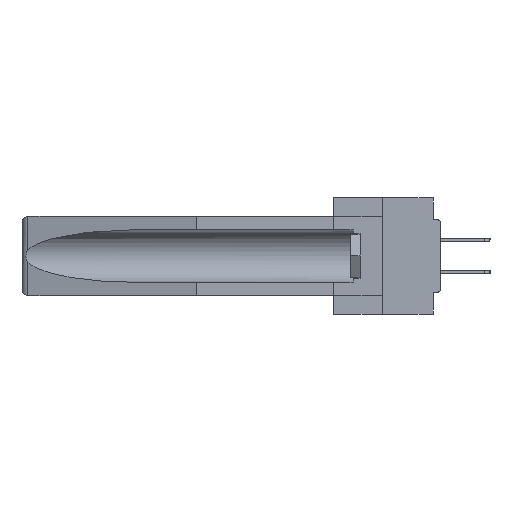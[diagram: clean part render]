
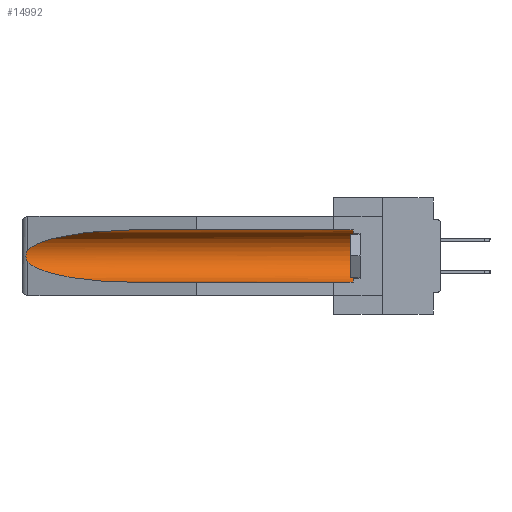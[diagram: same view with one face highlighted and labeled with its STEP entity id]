
A CAD part, left-side view. The second image highlights one B-rep face of the part: STEP entity #14992.
In plain terms, the highlighted cylindrical face has radius 2.857 mm (diameter 5.715 mm), a partial arc.
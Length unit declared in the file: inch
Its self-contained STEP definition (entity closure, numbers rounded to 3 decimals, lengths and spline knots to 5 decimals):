
#111 = VERTEX_POINT ( 'NONE', #24628 ) ;
#207 = VECTOR ( 'NONE', #23239, 39.37008 ) ;
#269 = CARTESIAN_POINT ( 'NONE',  ( 0.155, 1.07973, -0.284 ) ) ;
#1505 = LINE ( 'NONE', #4396, #2415 ) ;
#2100 = ORIENTED_EDGE ( 'NONE', *, *, #27193, .F. ) ;
#2415 = VECTOR ( 'NONE', #7474, 39.37008 ) ;
#3711 = CARTESIAN_POINT ( 'NONE',  ( 0.25451, 1.48313, -0.24835 ) ) ;
#3872 = ORIENTED_EDGE ( 'NONE', *, *, #9727, .T. ) ;
#4396 = CARTESIAN_POINT ( 'NONE',  ( 0.155, -0.30754, -0.059 ) ) ;
#4948 = CARTESIAN_POINT ( 'NONE',  ( 0.2675, 1.53308, -0.16763 ) ) ;
#5021 = VERTEX_POINT ( 'NONE', #32688 ) ;
#6171 = CYLINDRICAL_SURFACE ( 'NONE', #29870, 0.1125 ) ;
#6423 = CARTESIAN_POINT ( 'NONE',  ( 0.21114, 1.30732, -0.284 ) ) ;
#6682 = LINE ( 'NONE', #29462, #207 ) ;
#6717 = DIRECTION ( 'NONE',  ( 0., -1., 0. ) ) ;
#7474 = DIRECTION ( 'NONE',  ( 0., 1., 0. ) ) ;
#8298 = VERTEX_POINT ( 'NONE', #269 ) ;
#9727 = EDGE_CURVE ( 'NONE', #20303, #17446, #24305, .T. ) ;
#10373 = CARTESIAN_POINT ( 'NONE',  ( 0.26537, 1.52718, -0.19328 ) ) ;
#11486 = DIRECTION ( 'NONE',  ( 0., 0., 1. ) ) ;
#11732 = AXIS2_PLACEMENT_3D ( 'NONE', #24704, #6717, #22500 ) ;
#12064 = CARTESIAN_POINT ( 'NONE',  ( 0.155, 1.07973, -0.284 ) ) ;
#13337 = CARTESIAN_POINT ( 'NONE',  ( 0.26597, 1.52961, -0.15275 ) ) ;
#13363 = CARTESIAN_POINT ( 'NONE',  ( 0.21114, 1.30732, -0.059 ) ) ;
#13642 = CARTESIAN_POINT ( 'NONE',  ( 0.155, 0.126, -0.059 ) ) ;
#13966 = CARTESIAN_POINT ( 'NONE',  ( 0.26537, 1.52718, -0.19328 ) ) ;
#14992 = ADVANCED_FACE ( 'NONE', ( #31462 ), #6171, .F. ) ;
#15349 =( BOUNDED_CURVE ( )  B_SPLINE_CURVE ( 3, ( #18247, #13363, #36977, #19280 ),
 .UNSPECIFIED., .F., .F. ) 
 B_SPLINE_CURVE_WITH_KNOTS ( ( 4, 4 ),
 ( 4.71239, 6.08839 ),
 .UNSPECIFIED. ) 
 CURVE ( )  GEOMETRIC_REPRESENTATION_ITEM ( )  RATIONAL_B_SPLINE_CURVE ( ( 1., 0.848, 0.848, 1. ) ) 
 REPRESENTATION_ITEM ( '' )  );
#16535 = CARTESIAN_POINT ( 'NONE',  ( 0.26654, 1.53092, -0.15636 ) ) ;
#16571 = VERTEX_POINT ( 'NONE', #13642 ) ;
#17446 = VERTEX_POINT ( 'NONE', #13966 ) ;
#18247 = CARTESIAN_POINT ( 'NONE',  ( 0.155, 1.07973, -0.059 ) ) ;
#18946 = CIRCLE ( 'NONE', #11732, 0.1125 ) ;
#19280 = CARTESIAN_POINT ( 'NONE',  ( 0.26537, 1.52718, -0.14972 ) ) ;
#19889 = ORIENTED_EDGE ( 'NONE', *, *, #30012, .T. ) ;
#20303 = VERTEX_POINT ( 'NONE', #37683 ) ;
#21629 = EDGE_CURVE ( 'NONE', #16571, #5021, #1505, .T. ) ;
#22108 = CARTESIAN_POINT ( 'NONE',  ( 0.26597, 1.5296, -0.19026 ) ) ;
#22123 = EDGE_CURVE ( 'NONE', #111, #16571, #18946, .T. ) ;
#22500 = DIRECTION ( 'NONE',  ( 0., 0., 1. ) ) ;
#23239 = DIRECTION ( 'NONE',  ( 0., 1., 0. ) ) ;
#24218 = ORIENTED_EDGE ( 'NONE', *, *, #22123, .T. ) ;
#24305 = B_SPLINE_CURVE_WITH_KNOTS ( 'NONE', 3,
 ( #33830, #13337, #16535, #25014, #4948, #28263, #25388, #25138, #22108, #10373 ),
 .UNSPECIFIED., .F., .F.,
 ( 4, 2, 2, 2, 4 ),
 ( 0., 0.00029, 0.00058, 0.00087, 0.00117 ),
 .UNSPECIFIED. ) ;
#24628 = CARTESIAN_POINT ( 'NONE',  ( 0.155, 0.126, -0.284 ) ) ;
#24704 = CARTESIAN_POINT ( 'NONE',  ( 0.155, 0.126, -0.1715 ) ) ;
#25014 = CARTESIAN_POINT ( 'NONE',  ( 0.2673, 1.5327, -0.16383 ) ) ;
#25138 = CARTESIAN_POINT ( 'NONE',  ( 0.26655, 1.53094, -0.18657 ) ) ;
#25388 = CARTESIAN_POINT ( 'NONE',  ( 0.2673, 1.53269, -0.17917 ) ) ;
#26284 = DIRECTION ( 'NONE',  ( 0., 1., 0. ) ) ;
#27193 = EDGE_CURVE ( 'NONE', #111, #8298, #6682, .T. ) ;
#28263 = CARTESIAN_POINT ( 'NONE',  ( 0.2675, 1.53308, -0.17534 ) ) ;
#28827 = EDGE_LOOP ( 'NONE', ( #19889, #3872, #33713, #2100, #24218, #35631 ) ) ;
#29020 =( BOUNDED_CURVE ( )  B_SPLINE_CURVE ( 3, ( #32941, #3711, #6423, #12064 ),
 .UNSPECIFIED., .F., .F. ) 
 B_SPLINE_CURVE_WITH_KNOTS ( ( 4, 4 ),
 ( 0.1948, 1.5708 ),
 .UNSPECIFIED. ) 
 CURVE ( )  GEOMETRIC_REPRESENTATION_ITEM ( )  RATIONAL_B_SPLINE_CURVE ( ( 1., 0.848, 0.848, 1. ) ) 
 REPRESENTATION_ITEM ( '' )  );
#29462 = CARTESIAN_POINT ( 'NONE',  ( 0.155, -0.30754, -0.284 ) ) ;
#29522 = CARTESIAN_POINT ( 'NONE',  ( 0.155, -0.30754, -0.1715 ) ) ;
#29870 = AXIS2_PLACEMENT_3D ( 'NONE', #29522, #26284, #11486 ) ;
#30012 = EDGE_CURVE ( 'NONE', #5021, #20303, #15349, .T. ) ;
#31462 = FACE_OUTER_BOUND ( 'NONE', #28827, .T. ) ;
#32688 = CARTESIAN_POINT ( 'NONE',  ( 0.155, 1.07973, -0.059 ) ) ;
#32941 = CARTESIAN_POINT ( 'NONE',  ( 0.26537, 1.52718, -0.19328 ) ) ;
#33713 = ORIENTED_EDGE ( 'NONE', *, *, #38055, .T. ) ;
#33830 = CARTESIAN_POINT ( 'NONE',  ( 0.26537, 1.52718, -0.14972 ) ) ;
#35631 = ORIENTED_EDGE ( 'NONE', *, *, #21629, .T. ) ;
#36977 = CARTESIAN_POINT ( 'NONE',  ( 0.25451, 1.48313, -0.09465 ) ) ;
#37683 = CARTESIAN_POINT ( 'NONE',  ( 0.26537, 1.52718, -0.14972 ) ) ;
#38055 = EDGE_CURVE ( 'NONE', #17446, #8298, #29020, .T. ) ;
